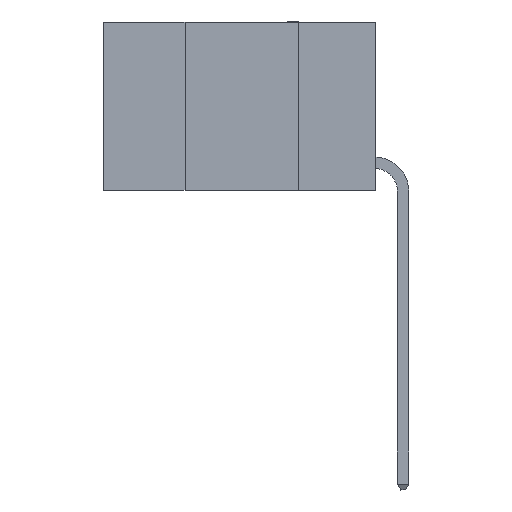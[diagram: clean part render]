
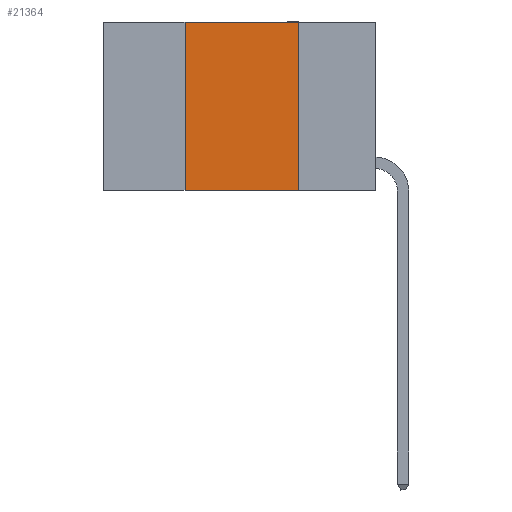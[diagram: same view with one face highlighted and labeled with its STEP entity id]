
A CAD part, left-side view. The second image highlights one B-rep face of the part: STEP entity #21364.
In plain terms, the highlighted planar face has unit normal (-1, 0, 0).
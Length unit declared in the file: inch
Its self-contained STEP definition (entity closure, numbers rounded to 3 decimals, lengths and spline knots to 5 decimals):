
#258 = EDGE_CURVE ( 'NONE', #14419, #7220, #9642, .T. ) ;
#1377 = DIRECTION ( 'NONE',  ( 0., 0., -1. ) ) ;
#1428 = VECTOR ( 'NONE', #2429, 39.37008 ) ;
#2429 = DIRECTION ( 'NONE',  ( 0., 0., -1. ) ) ;
#2490 = EDGE_CURVE ( 'NONE', #7220, #12279, #20659, .T. ) ;
#2530 = ORIENTED_EDGE ( 'NONE', *, *, #258, .F. ) ;
#2667 = EDGE_CURVE ( 'NONE', #14419, #6102, #6313, .T. ) ;
#3975 = VECTOR ( 'NONE', #11378, 39.37008 ) ;
#4142 = CARTESIAN_POINT ( 'NONE',  ( 0., 0.17, 0. ) ) ;
#4684 = EDGE_LOOP ( 'NONE', ( #7111, #6269, #2530, #5063 ) ) ;
#5063 = ORIENTED_EDGE ( 'NONE', *, *, #2667, .T. ) ;
#5334 = CARTESIAN_POINT ( 'NONE',  ( 0., 0.17, 0. ) ) ;
#5543 = CARTESIAN_POINT ( 'NONE',  ( 0., 0.6, 0. ) ) ;
#5799 = CARTESIAN_POINT ( 'NONE',  ( 0., 0.42, 0. ) ) ;
#6102 = VERTEX_POINT ( 'NONE', #9261 ) ;
#6269 = ORIENTED_EDGE ( 'NONE', *, *, #2490, .F. ) ;
#6313 = LINE ( 'NONE', #21560, #3975 ) ;
#7111 = ORIENTED_EDGE ( 'NONE', *, *, #11498, .F. ) ;
#7220 = VERTEX_POINT ( 'NONE', #16271 ) ;
#7565 = AXIS2_PLACEMENT_3D ( 'NONE', #13191, #16406, #1377 ) ;
#7903 = PLANE ( 'NONE',  #7565 ) ;
#9261 = CARTESIAN_POINT ( 'NONE',  ( 0., 0.17, -0.37 ) ) ;
#9642 = LINE ( 'NONE', #5799, #18024 ) ;
#9781 = FACE_OUTER_BOUND ( 'NONE', #4684, .T. ) ;
#10831 = LINE ( 'NONE', #5334, #1428 ) ;
#11378 = DIRECTION ( 'NONE',  ( 0., -1., 0. ) ) ;
#11498 = EDGE_CURVE ( 'NONE', #12279, #6102, #10831, .T. ) ;
#12254 = DIRECTION ( 'NONE',  ( 0., -1., 0. ) ) ;
#12279 = VERTEX_POINT ( 'NONE', #4142 ) ;
#13191 = CARTESIAN_POINT ( 'NONE',  ( 0., 0.6, 0. ) ) ;
#14419 = VERTEX_POINT ( 'NONE', #19324 ) ;
#16055 = DIRECTION ( 'NONE',  ( 0., 0., 1. ) ) ;
#16271 = CARTESIAN_POINT ( 'NONE',  ( 0., 0.42, 0. ) ) ;
#16406 = DIRECTION ( 'NONE',  ( 1., 0., 0. ) ) ;
#18024 = VECTOR ( 'NONE', #16055, 39.37008 ) ;
#19324 = CARTESIAN_POINT ( 'NONE',  ( 0., 0.42, -0.37 ) ) ;
#19673 = VECTOR ( 'NONE', #12254, 39.37008 ) ;
#20659 = LINE ( 'NONE', #5543, #19673 ) ;
#21364 = ADVANCED_FACE ( 'NONE', ( #9781 ), #7903, .F. ) ;
#21560 = CARTESIAN_POINT ( 'NONE',  ( 0., 0.6, -0.37 ) ) ;
